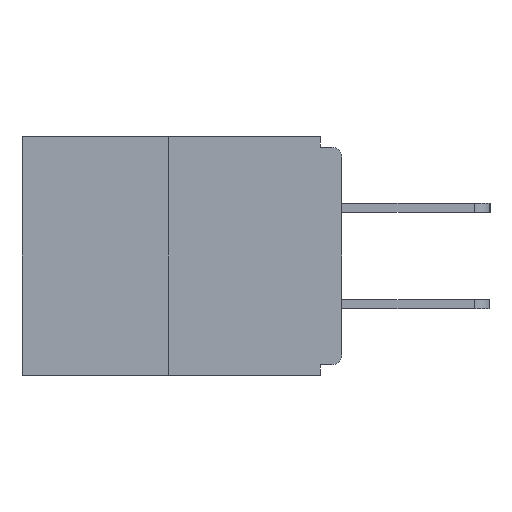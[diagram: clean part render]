
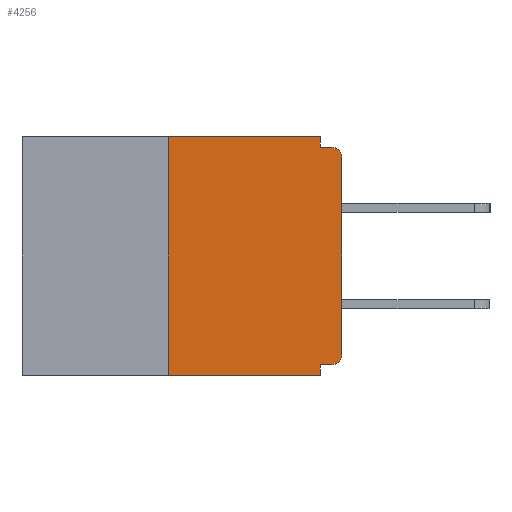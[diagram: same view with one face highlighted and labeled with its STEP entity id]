
A CAD part, left-side view. The second image highlights one B-rep face of the part: STEP entity #4256.
In plain terms, the highlighted planar face has unit normal (-1, 0, 0).
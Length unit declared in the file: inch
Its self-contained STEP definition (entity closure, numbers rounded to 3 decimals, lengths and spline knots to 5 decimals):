
#25 = CARTESIAN_POINT ( 'NONE',  ( 0., 0.25, -0.343 ) ) ;
#328 = DIRECTION ( 'NONE',  ( 0., 0., -1. ) ) ;
#373 = VERTEX_POINT ( 'NONE', #930 ) ;
#510 = EDGE_LOOP ( 'NONE', ( #7819, #2381, #1848, #13323, #7453, #1111, #9976, #5351, #1161, #2847 ) ) ;
#882 = CARTESIAN_POINT ( 'NONE',  ( 0., 0., -0.03 ) ) ;
#930 = CARTESIAN_POINT ( 'NONE',  ( 0., 0.25, 0. ) ) ;
#1111 = ORIENTED_EDGE ( 'NONE', *, *, #8801, .T. ) ;
#1144 = EDGE_CURVE ( 'NONE', #14052, #3665, #10006, .T. ) ;
#1161 = ORIENTED_EDGE ( 'NONE', *, *, #5610, .F. ) ;
#1615 = VECTOR ( 'NONE', #328, 39.37008 ) ;
#1657 = AXIS2_PLACEMENT_3D ( 'NONE', #1659, #9096, #5384 ) ;
#1659 = CARTESIAN_POINT ( 'NONE',  ( 0., 0.015, -0.313 ) ) ;
#1667 = VERTEX_POINT ( 'NONE', #8691 ) ;
#1692 = VECTOR ( 'NONE', #12297, 39.37008 ) ;
#1848 = ORIENTED_EDGE ( 'NONE', *, *, #14366, .T. ) ;
#1865 = CARTESIAN_POINT ( 'NONE',  ( 0., 0.031, -0.015 ) ) ;
#1981 = DIRECTION ( 'NONE',  ( 0., -1., 0. ) ) ;
#2264 = DIRECTION ( 'NONE',  ( 0., 0., -1. ) ) ;
#2381 = ORIENTED_EDGE ( 'NONE', *, *, #2505, .F. ) ;
#2414 = VERTEX_POINT ( 'NONE', #882 ) ;
#2505 = EDGE_CURVE ( 'NONE', #7591, #373, #13585, .T. ) ;
#2847 = ORIENTED_EDGE ( 'NONE', *, *, #4136, .F. ) ;
#3505 = CARTESIAN_POINT ( 'NONE',  ( 0., 0.46, 0. ) ) ;
#3665 = VERTEX_POINT ( 'NONE', #4401 ) ;
#3776 = EDGE_CURVE ( 'NONE', #2414, #8285, #9919, .T. ) ;
#3872 = VECTOR ( 'NONE', #1981, 39.37008 ) ;
#4136 = EDGE_CURVE ( 'NONE', #5708, #8321, #6480, .T. ) ;
#4239 = AXIS2_PLACEMENT_3D ( 'NONE', #10614, #14668, #10840 ) ;
#4256 = ADVANCED_FACE ( 'NONE', ( #10747 ), #9626, .F. ) ;
#4401 = CARTESIAN_POINT ( 'NONE',  ( 0., 0.031, -0.328 ) ) ;
#4473 = AXIS2_PLACEMENT_3D ( 'NONE', #13364, #8420, #2264 ) ;
#4909 = CARTESIAN_POINT ( 'NONE',  ( 0., 0., -0.328 ) ) ;
#5058 = CARTESIAN_POINT ( 'NONE',  ( 0., 0., -0.313 ) ) ;
#5074 = DIRECTION ( 'NONE',  ( 0., 1., 0. ) ) ;
#5351 = ORIENTED_EDGE ( 'NONE', *, *, #3776, .T. ) ;
#5384 = DIRECTION ( 'NONE',  ( 0., 0., -1. ) ) ;
#5610 = EDGE_CURVE ( 'NONE', #8321, #8285, #5793, .T. ) ;
#5708 = VERTEX_POINT ( 'NONE', #12107 ) ;
#5717 = CARTESIAN_POINT ( 'NONE',  ( 0., 0., -0.015 ) ) ;
#5738 = CARTESIAN_POINT ( 'NONE',  ( 0., 0.015, -0.015 ) ) ;
#5762 = VERTEX_POINT ( 'NONE', #5058 ) ;
#5793 = LINE ( 'NONE', #5717, #9061 ) ;
#6044 = EDGE_CURVE ( 'NONE', #373, #5708, #8198, .T. ) ;
#6124 = CARTESIAN_POINT ( 'NONE',  ( 0., 0.25, 0. ) ) ;
#6245 = DIRECTION ( 'NONE',  ( 0., 0., -1. ) ) ;
#6480 = LINE ( 'NONE', #11417, #1615 ) ;
#7102 = VECTOR ( 'NONE', #5074, 39.37008 ) ;
#7453 = ORIENTED_EDGE ( 'NONE', *, *, #1144, .F. ) ;
#7591 = VERTEX_POINT ( 'NONE', #25 ) ;
#7819 = ORIENTED_EDGE ( 'NONE', *, *, #6044, .F. ) ;
#8198 = LINE ( 'NONE', #3505, #3872 ) ;
#8285 = VERTEX_POINT ( 'NONE', #5738 ) ;
#8321 = VERTEX_POINT ( 'NONE', #1865 ) ;
#8420 = DIRECTION ( 'NONE',  ( 1., 0., 0. ) ) ;
#8475 = VECTOR ( 'NONE', #11288, 39.37008 ) ;
#8691 = CARTESIAN_POINT ( 'NONE',  ( 0., 0.031, -0.343 ) ) ;
#8801 = EDGE_CURVE ( 'NONE', #14052, #5762, #8882, .T. ) ;
#8882 = CIRCLE ( 'NONE', #1657, 0.015 ) ;
#9061 = VECTOR ( 'NONE', #9593, 39.37008 ) ;
#9096 = DIRECTION ( 'NONE',  ( -1., 0., 0. ) ) ;
#9593 = DIRECTION ( 'NONE',  ( 0., -1., 0. ) ) ;
#9626 = PLANE ( 'NONE',  #4473 ) ;
#9737 = CARTESIAN_POINT ( 'NONE',  ( 0., 0.015, -0.328 ) ) ;
#9774 = CARTESIAN_POINT ( 'NONE',  ( 0., 0.46, -0.343 ) ) ;
#9845 = DIRECTION ( 'NONE',  ( 0., 0., 1. ) ) ;
#9919 = CIRCLE ( 'NONE', #4239, 0.015 ) ;
#9976 = ORIENTED_EDGE ( 'NONE', *, *, #10570, .T. ) ;
#10006 = LINE ( 'NONE', #4909, #7102 ) ;
#10381 = EDGE_CURVE ( 'NONE', #3665, #1667, #13700, .T. ) ;
#10570 = EDGE_CURVE ( 'NONE', #5762, #2414, #11758, .T. ) ;
#10614 = CARTESIAN_POINT ( 'NONE',  ( 0., 0.015, -0.03 ) ) ;
#10747 = FACE_OUTER_BOUND ( 'NONE', #510, .T. ) ;
#10840 = DIRECTION ( 'NONE',  ( 0., 0., -1. ) ) ;
#11288 = DIRECTION ( 'NONE',  ( 0., 0., 1. ) ) ;
#11417 = CARTESIAN_POINT ( 'NONE',  ( 0., 0.031, 0. ) ) ;
#11758 = LINE ( 'NONE', #12978, #8475 ) ;
#12107 = CARTESIAN_POINT ( 'NONE',  ( 0., 0.031, 0. ) ) ;
#12205 = LINE ( 'NONE', #9774, #1692 ) ;
#12297 = DIRECTION ( 'NONE',  ( 0., -1., 0. ) ) ;
#12857 = VECTOR ( 'NONE', #9845, 39.37008 ) ;
#12877 = VECTOR ( 'NONE', #6245, 39.37008 ) ;
#12978 = CARTESIAN_POINT ( 'NONE',  ( 0., 0., 0. ) ) ;
#13323 = ORIENTED_EDGE ( 'NONE', *, *, #10381, .F. ) ;
#13364 = CARTESIAN_POINT ( 'NONE',  ( 0., 0.46, 0. ) ) ;
#13585 = LINE ( 'NONE', #6124, #12857 ) ;
#13625 = CARTESIAN_POINT ( 'NONE',  ( 0., 0.031, -0.343 ) ) ;
#13700 = LINE ( 'NONE', #13625, #12877 ) ;
#14052 = VERTEX_POINT ( 'NONE', #9737 ) ;
#14366 = EDGE_CURVE ( 'NONE', #7591, #1667, #12205, .T. ) ;
#14668 = DIRECTION ( 'NONE',  ( -1., 0., 0. ) ) ;
